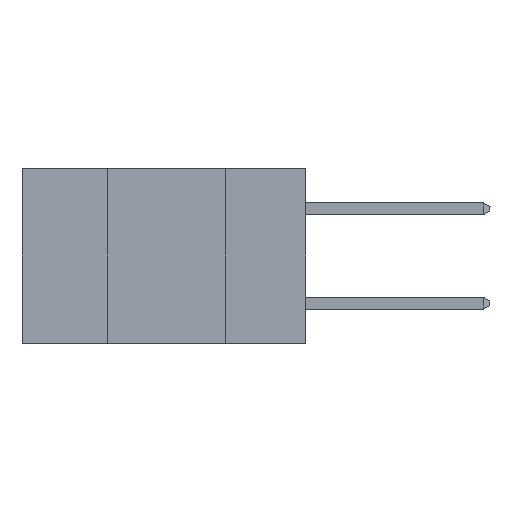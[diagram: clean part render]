
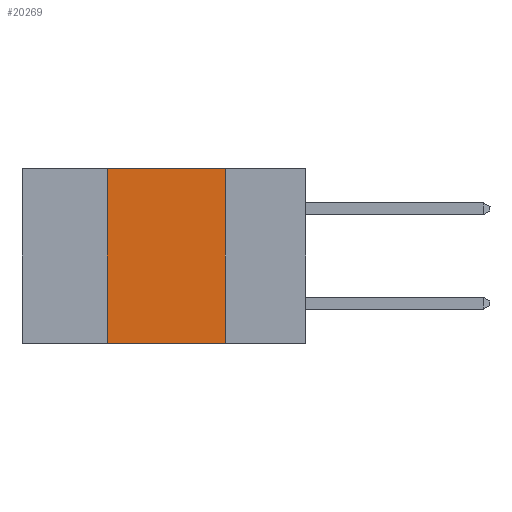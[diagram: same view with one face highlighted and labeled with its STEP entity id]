
A CAD part, left-side view. The second image highlights one B-rep face of the part: STEP entity #20269.
In plain terms, the highlighted planar face has unit normal (-1, 0, 0).
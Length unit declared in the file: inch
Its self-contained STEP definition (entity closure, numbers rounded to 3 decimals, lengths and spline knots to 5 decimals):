
#142 = CARTESIAN_POINT ( 'NONE',  ( 0., 0.42, -0.37 ) ) ;
#945 = LINE ( 'NONE', #12357, #9610 ) ;
#1317 = LINE ( 'NONE', #22538, #22445 ) ;
#1417 = CARTESIAN_POINT ( 'NONE',  ( 0., 0.42, 0. ) ) ;
#1692 = DIRECTION ( 'NONE',  ( 0., -1., 0. ) ) ;
#3211 = ORIENTED_EDGE ( 'NONE', *, *, #7845, .T. ) ;
#3660 = DIRECTION ( 'NONE',  ( 0., 0., 1. ) ) ;
#3742 = CARTESIAN_POINT ( 'NONE',  ( 0., 0.17, 0. ) ) ;
#4518 = DIRECTION ( 'NONE',  ( 1., 0., 0. ) ) ;
#5062 = VERTEX_POINT ( 'NONE', #17409 ) ;
#5289 = DIRECTION ( 'NONE',  ( 0., 0., -1. ) ) ;
#7698 = ORIENTED_EDGE ( 'NONE', *, *, #12321, .F. ) ;
#7845 = EDGE_CURVE ( 'NONE', #16822, #10946, #945, .T. ) ;
#8138 = CARTESIAN_POINT ( 'NONE',  ( 0., 0.17, -0.37 ) ) ;
#8360 = LINE ( 'NONE', #17990, #14240 ) ;
#9610 = VECTOR ( 'NONE', #1692, 39.37008 ) ;
#10946 = VERTEX_POINT ( 'NONE', #8138 ) ;
#11433 = EDGE_CURVE ( 'NONE', #5062, #10946, #22801, .T. ) ;
#11852 = DIRECTION ( 'NONE',  ( 0., 0., -1. ) ) ;
#12221 = VERTEX_POINT ( 'NONE', #1417 ) ;
#12233 = AXIS2_PLACEMENT_3D ( 'NONE', #22414, #4518, #11852 ) ;
#12321 = EDGE_CURVE ( 'NONE', #12221, #5062, #1317, .T. ) ;
#12357 = CARTESIAN_POINT ( 'NONE',  ( 0., 0.6, -0.37 ) ) ;
#14240 = VECTOR ( 'NONE', #3660, 39.37008 ) ;
#15254 = DIRECTION ( 'NONE',  ( 0., -1., 0. ) ) ;
#16822 = VERTEX_POINT ( 'NONE', #142 ) ;
#16928 = PLANE ( 'NONE',  #12233 ) ;
#17409 = CARTESIAN_POINT ( 'NONE',  ( 0., 0.17, 0. ) ) ;
#17990 = CARTESIAN_POINT ( 'NONE',  ( 0., 0.42, 0. ) ) ;
#19552 = FACE_OUTER_BOUND ( 'NONE', #23020, .T. ) ;
#20269 = ADVANCED_FACE ( 'NONE', ( #19552 ), #16928, .F. ) ;
#20497 = EDGE_CURVE ( 'NONE', #16822, #12221, #8360, .T. ) ;
#21318 = ORIENTED_EDGE ( 'NONE', *, *, #20497, .F. ) ;
#21687 = VECTOR ( 'NONE', #5289, 39.37008 ) ;
#22369 = ORIENTED_EDGE ( 'NONE', *, *, #11433, .F. ) ;
#22414 = CARTESIAN_POINT ( 'NONE',  ( 0., 0.6, 0. ) ) ;
#22445 = VECTOR ( 'NONE', #15254, 39.37008 ) ;
#22538 = CARTESIAN_POINT ( 'NONE',  ( 0., 0.6, 0. ) ) ;
#22801 = LINE ( 'NONE', #3742, #21687 ) ;
#23020 = EDGE_LOOP ( 'NONE', ( #22369, #7698, #21318, #3211 ) ) ;
